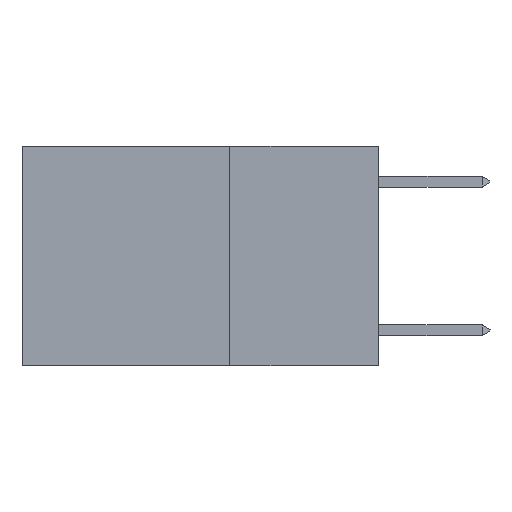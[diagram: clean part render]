
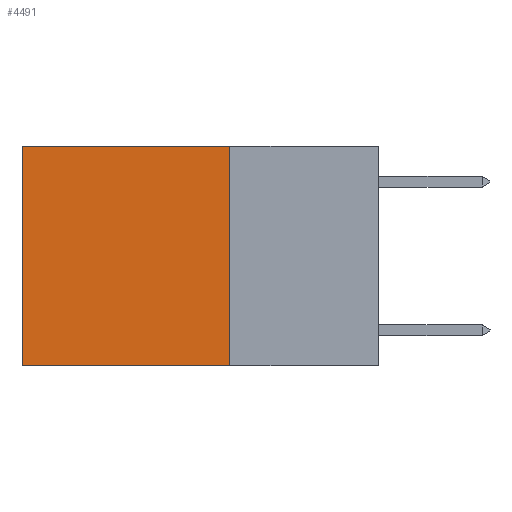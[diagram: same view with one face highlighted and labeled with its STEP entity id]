
A CAD part, left-side view. The second image highlights one B-rep face of the part: STEP entity #4491.
In plain terms, the highlighted planar face has unit normal (-1, 0, 0).
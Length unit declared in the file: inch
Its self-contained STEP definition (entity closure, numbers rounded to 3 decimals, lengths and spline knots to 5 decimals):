
#522 = VERTEX_POINT ( 'NONE', #9218 ) ;
#915 = AXIS2_PLACEMENT_3D ( 'NONE', #4816, #3992, #3940 ) ;
#1597 = CARTESIAN_POINT ( 'NONE',  ( 0.2625, 0.25, 0. ) ) ;
#1701 = VECTOR ( 'NONE', #3133, 39.37008 ) ;
#1838 = LINE ( 'NONE', #1597, #5908 ) ;
#1906 = ORIENTED_EDGE ( 'NONE', *, *, #9591, .T. ) ;
#2369 = CARTESIAN_POINT ( 'NONE',  ( 0.2625, 0.25, 0. ) ) ;
#2471 = DIRECTION ( 'NONE',  ( 0., 0., -1. ) ) ;
#2642 = CARTESIAN_POINT ( 'NONE',  ( 0.2625, 0.6, 0. ) ) ;
#2732 = CARTESIAN_POINT ( 'NONE',  ( 0.2625, 0.25, -0.37 ) ) ;
#2790 = ORIENTED_EDGE ( 'NONE', *, *, #7186, .F. ) ;
#2822 = DIRECTION ( 'NONE',  ( 0., 1., 0. ) ) ;
#2929 = VERTEX_POINT ( 'NONE', #9700 ) ;
#2947 = ORIENTED_EDGE ( 'NONE', *, *, #9466, .F. ) ;
#3133 = DIRECTION ( 'NONE',  ( 0., 0., -1. ) ) ;
#3940 = DIRECTION ( 'NONE',  ( 0., 0., -1. ) ) ;
#3992 = DIRECTION ( 'NONE',  ( 1., 0., 0. ) ) ;
#4040 = PLANE ( 'NONE',  #915 ) ;
#4151 = ORIENTED_EDGE ( 'NONE', *, *, #8705, .T. ) ;
#4176 = EDGE_LOOP ( 'NONE', ( #1906, #2790, #2947, #4151 ) ) ;
#4376 = FACE_OUTER_BOUND ( 'NONE', #4176, .T. ) ;
#4491 = ADVANCED_FACE ( 'NONE', ( #4376 ), #4040, .F. ) ;
#4731 = LINE ( 'NONE', #8585, #8412 ) ;
#4816 = CARTESIAN_POINT ( 'NONE',  ( 0.2625, 0.25, 0. ) ) ;
#5908 = VECTOR ( 'NONE', #7074, 39.37008 ) ;
#6898 = VECTOR ( 'NONE', #2822, 39.37008 ) ;
#7074 = DIRECTION ( 'NONE',  ( 0., 1., 0. ) ) ;
#7117 = LINE ( 'NONE', #7531, #6898 ) ;
#7186 = EDGE_CURVE ( 'NONE', #9141, #2929, #7117, .T. ) ;
#7531 = CARTESIAN_POINT ( 'NONE',  ( 0.2625, 0.25, -0.37 ) ) ;
#7828 = VERTEX_POINT ( 'NONE', #2642 ) ;
#7859 = LINE ( 'NONE', #2369, #1701 ) ;
#8412 = VECTOR ( 'NONE', #2471, 39.37008 ) ;
#8585 = CARTESIAN_POINT ( 'NONE',  ( 0.2625, 0.6, 0. ) ) ;
#8705 = EDGE_CURVE ( 'NONE', #522, #7828, #1838, .T. ) ;
#9141 = VERTEX_POINT ( 'NONE', #2732 ) ;
#9218 = CARTESIAN_POINT ( 'NONE',  ( 0.2625, 0.25, 0. ) ) ;
#9466 = EDGE_CURVE ( 'NONE', #522, #9141, #7859, .T. ) ;
#9591 = EDGE_CURVE ( 'NONE', #7828, #2929, #4731, .T. ) ;
#9700 = CARTESIAN_POINT ( 'NONE',  ( 0.2625, 0.6, -0.37 ) ) ;
